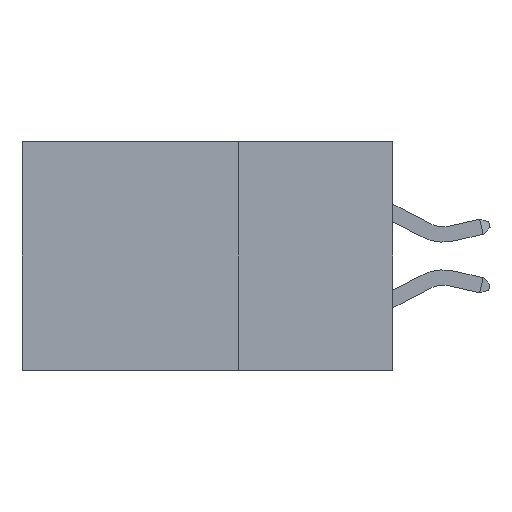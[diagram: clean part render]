
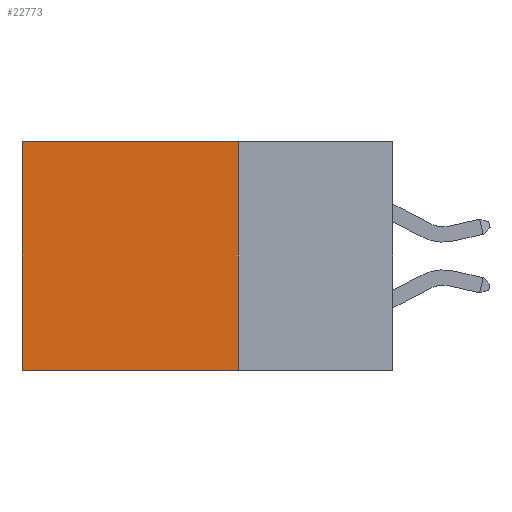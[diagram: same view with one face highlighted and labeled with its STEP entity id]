
A CAD part, left-side view. The second image highlights one B-rep face of the part: STEP entity #22773.
In plain terms, the highlighted planar face has unit normal (-1, 0, 0).
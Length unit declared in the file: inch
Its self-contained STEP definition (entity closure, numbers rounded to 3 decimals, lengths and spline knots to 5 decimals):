
#455 = DIRECTION ( 'NONE',  ( 0., 0., -1. ) ) ;
#1191 = CARTESIAN_POINT ( 'NONE',  ( 0.2875, 0.6, 0. ) ) ;
#3067 = CARTESIAN_POINT ( 'NONE',  ( 0.2875, 0.6, 0. ) ) ;
#3776 = PLANE ( 'NONE',  #12843 ) ;
#3991 = VECTOR ( 'NONE', #26973, 39.37008 ) ;
#4319 = LINE ( 'NONE', #15937, #3991 ) ;
#4407 = VERTEX_POINT ( 'NONE', #35373 ) ;
#5253 = EDGE_CURVE ( 'NONE', #13742, #29444, #13360, .T. ) ;
#5439 = ORIENTED_EDGE ( 'NONE', *, *, #27092, .T. ) ;
#7361 = EDGE_CURVE ( 'NONE', #4407, #29444, #4319, .T. ) ;
#8917 = LINE ( 'NONE', #20510, #28145 ) ;
#9513 = FACE_OUTER_BOUND ( 'NONE', #14726, .T. ) ;
#10061 = VERTEX_POINT ( 'NONE', #22468 ) ;
#10730 = ORIENTED_EDGE ( 'NONE', *, *, #7361, .F. ) ;
#12633 = CARTESIAN_POINT ( 'NONE',  ( 0.2875, 0.6, -0.37 ) ) ;
#12843 = AXIS2_PLACEMENT_3D ( 'NONE', #15215, #30202, #33050 ) ;
#13360 = LINE ( 'NONE', #1191, #34947 ) ;
#13742 = VERTEX_POINT ( 'NONE', #3067 ) ;
#14726 = EDGE_LOOP ( 'NONE', ( #22222, #10730, #31777, #5439 ) ) ;
#15215 = CARTESIAN_POINT ( 'NONE',  ( 0.2875, 0.25, 0. ) ) ;
#15937 = CARTESIAN_POINT ( 'NONE',  ( 0.2875, 0.25, -0.37 ) ) ;
#19240 = DIRECTION ( 'NONE',  ( 0., 0., -1. ) ) ;
#20510 = CARTESIAN_POINT ( 'NONE',  ( 0.2875, 0.25, 0. ) ) ;
#21161 = LINE ( 'NONE', #32191, #31828 ) ;
#22222 = ORIENTED_EDGE ( 'NONE', *, *, #5253, .T. ) ;
#22468 = CARTESIAN_POINT ( 'NONE',  ( 0.2875, 0.25, 0. ) ) ;
#22773 = ADVANCED_FACE ( 'NONE', ( #9513 ), #3776, .F. ) ;
#26238 = EDGE_CURVE ( 'NONE', #10061, #4407, #21161, .T. ) ;
#26973 = DIRECTION ( 'NONE',  ( 0., 1., 0. ) ) ;
#27092 = EDGE_CURVE ( 'NONE', #10061, #13742, #8917, .T. ) ;
#28145 = VECTOR ( 'NONE', #32090, 39.37008 ) ;
#29444 = VERTEX_POINT ( 'NONE', #12633 ) ;
#30202 = DIRECTION ( 'NONE',  ( 1., 0., 0. ) ) ;
#31777 = ORIENTED_EDGE ( 'NONE', *, *, #26238, .F. ) ;
#31828 = VECTOR ( 'NONE', #455, 39.37008 ) ;
#32090 = DIRECTION ( 'NONE',  ( 0., 1., 0. ) ) ;
#32191 = CARTESIAN_POINT ( 'NONE',  ( 0.2875, 0.25, 0. ) ) ;
#33050 = DIRECTION ( 'NONE',  ( 0., 0., -1. ) ) ;
#34947 = VECTOR ( 'NONE', #19240, 39.37008 ) ;
#35373 = CARTESIAN_POINT ( 'NONE',  ( 0.2875, 0.25, -0.37 ) ) ;
